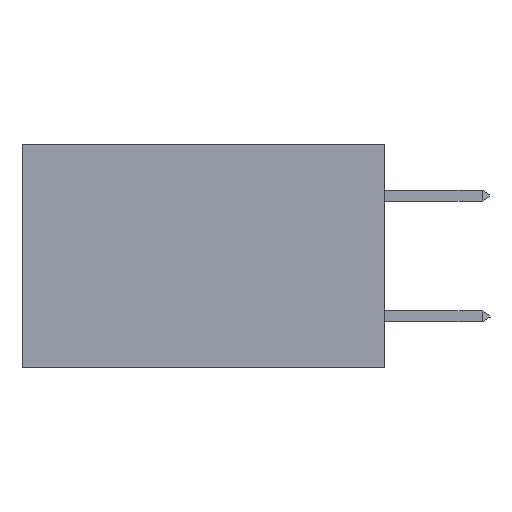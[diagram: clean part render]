
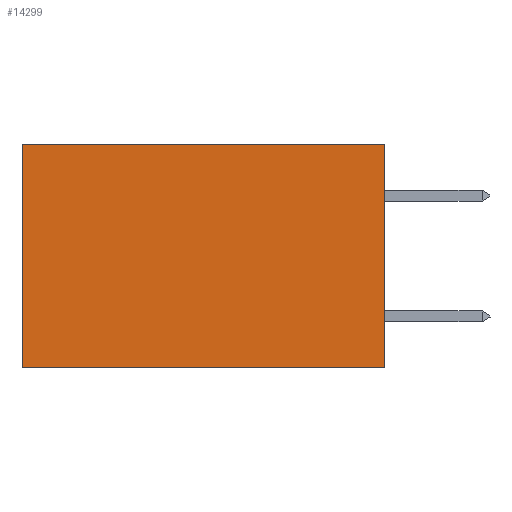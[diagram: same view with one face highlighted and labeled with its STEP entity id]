
A CAD part, left-side view. The second image highlights one B-rep face of the part: STEP entity #14299.
In plain terms, the highlighted planar face has unit normal (-1, 0, 0).
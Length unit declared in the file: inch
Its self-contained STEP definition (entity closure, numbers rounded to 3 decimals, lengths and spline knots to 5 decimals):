
#334 = ORIENTED_EDGE ( 'NONE', *, *, #17587, .F. ) ;
#499 = VERTEX_POINT ( 'NONE', #5244 ) ;
#1098 = EDGE_LOOP ( 'NONE', ( #12458, #14049, #334, #2710 ) ) ;
#2710 = ORIENTED_EDGE ( 'NONE', *, *, #17327, .T. ) ;
#2928 = PLANE ( 'NONE',  #10572 ) ;
#4806 = LINE ( 'NONE', #18654, #16562 ) ;
#5244 = CARTESIAN_POINT ( 'NONE',  ( 0.2875, 0.6, -0.37 ) ) ;
#5856 = CARTESIAN_POINT ( 'NONE',  ( 0.2875, 0.6, 0. ) ) ;
#5949 = FACE_OUTER_BOUND ( 'NONE', #1098, .T. ) ;
#5981 = CARTESIAN_POINT ( 'NONE',  ( 0.2875, 0., 0. ) ) ;
#6004 = DIRECTION ( 'NONE',  ( 0., 0., -1. ) ) ;
#6784 = VECTOR ( 'NONE', #15188, 39.37008 ) ;
#7524 = VECTOR ( 'NONE', #19181, 39.37008 ) ;
#7560 = VERTEX_POINT ( 'NONE', #19070 ) ;
#7956 = DIRECTION ( 'NONE',  ( 0., 1., 0. ) ) ;
#8657 = CARTESIAN_POINT ( 'NONE',  ( 0.2875, 0., -0.37 ) ) ;
#9202 = VERTEX_POINT ( 'NONE', #8657 ) ;
#9626 = LINE ( 'NONE', #5856, #13722 ) ;
#9694 = VERTEX_POINT ( 'NONE', #12875 ) ;
#10572 = AXIS2_PLACEMENT_3D ( 'NONE', #10609, #15210, #6004 ) ;
#10609 = CARTESIAN_POINT ( 'NONE',  ( 0.2875, 0., 0. ) ) ;
#11404 = LINE ( 'NONE', #5981, #6784 ) ;
#12458 = ORIENTED_EDGE ( 'NONE', *, *, #19702, .T. ) ;
#12875 = CARTESIAN_POINT ( 'NONE',  ( 0.2875, 0., 0. ) ) ;
#13722 = VECTOR ( 'NONE', #16578, 39.37008 ) ;
#14049 = ORIENTED_EDGE ( 'NONE', *, *, #19023, .F. ) ;
#14299 = ADVANCED_FACE ( 'NONE', ( #5949 ), #2928, .F. ) ;
#14612 = CARTESIAN_POINT ( 'NONE',  ( 0.2875, 0., 0. ) ) ;
#15188 = DIRECTION ( 'NONE',  ( 0., 0., -1. ) ) ;
#15210 = DIRECTION ( 'NONE',  ( 1., 0., 0. ) ) ;
#16562 = VECTOR ( 'NONE', #7956, 39.37008 ) ;
#16578 = DIRECTION ( 'NONE',  ( 0., 0., -1. ) ) ;
#17327 = EDGE_CURVE ( 'NONE', #9694, #7560, #19739, .T. ) ;
#17587 = EDGE_CURVE ( 'NONE', #9694, #9202, #11404, .T. ) ;
#18654 = CARTESIAN_POINT ( 'NONE',  ( 0.2875, 0., -0.37 ) ) ;
#19023 = EDGE_CURVE ( 'NONE', #9202, #499, #4806, .T. ) ;
#19070 = CARTESIAN_POINT ( 'NONE',  ( 0.2875, 0.6, 0. ) ) ;
#19181 = DIRECTION ( 'NONE',  ( 0., 1., 0. ) ) ;
#19702 = EDGE_CURVE ( 'NONE', #7560, #499, #9626, .T. ) ;
#19739 = LINE ( 'NONE', #14612, #7524 ) ;
